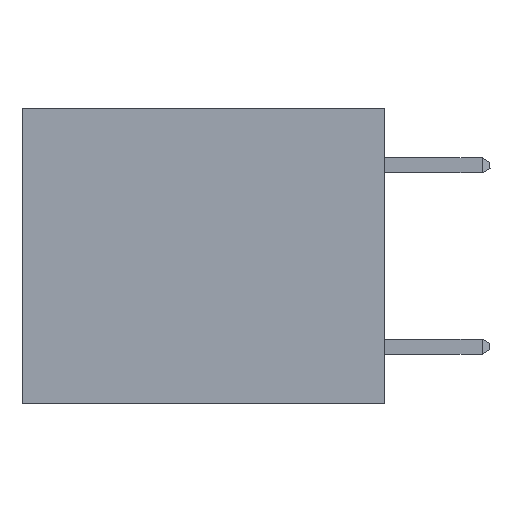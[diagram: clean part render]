
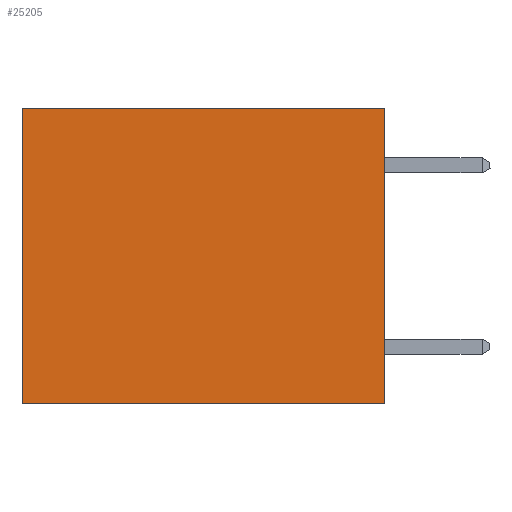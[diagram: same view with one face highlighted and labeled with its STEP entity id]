
A CAD part, left-side view. The second image highlights one B-rep face of the part: STEP entity #25205.
In plain terms, the highlighted planar face has unit normal (-1, 0, 0).
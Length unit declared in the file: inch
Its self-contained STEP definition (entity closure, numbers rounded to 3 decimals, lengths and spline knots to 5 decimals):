
#821 = LINE ( 'NONE', #17745, #24701 ) ;
#902 = EDGE_CURVE ( 'NONE', #22420, #20149, #2987, .T. ) ;
#1377 = DIRECTION ( 'NONE',  ( 0., 0., -1. ) ) ;
#2313 = VERTEX_POINT ( 'NONE', #26707 ) ;
#2987 = LINE ( 'NONE', #20899, #4164 ) ;
#4164 = VECTOR ( 'NONE', #8622, 39.37008 ) ;
#4547 = ORIENTED_EDGE ( 'NONE', *, *, #7767, .F. ) ;
#4949 = DIRECTION ( 'NONE',  ( 0., 1., 0. ) ) ;
#5919 = EDGE_LOOP ( 'NONE', ( #26563, #4547, #26533, #12764 ) ) ;
#7767 = EDGE_CURVE ( 'NONE', #22263, #20149, #821, .T. ) ;
#8622 = DIRECTION ( 'NONE',  ( 0., 0., -1. ) ) ;
#8946 = DIRECTION ( 'NONE',  ( 1., 0., 0. ) ) ;
#11538 = PLANE ( 'NONE',  #18131 ) ;
#12523 = CARTESIAN_POINT ( 'NONE',  ( 0.3165, 0.6, -0.49 ) ) ;
#12764 = ORIENTED_EDGE ( 'NONE', *, *, #16575, .T. ) ;
#15285 = VECTOR ( 'NONE', #17330, 39.37008 ) ;
#15567 = CARTESIAN_POINT ( 'NONE',  ( 0.3165, 0.6, 0. ) ) ;
#16575 = EDGE_CURVE ( 'NONE', #2313, #22420, #24248, .T. ) ;
#17330 = DIRECTION ( 'NONE',  ( 0., 0., -1. ) ) ;
#17742 = VECTOR ( 'NONE', #4949, 39.37008 ) ;
#17745 = CARTESIAN_POINT ( 'NONE',  ( 0.3165, 0., -0.49 ) ) ;
#18131 = AXIS2_PLACEMENT_3D ( 'NONE', #23652, #8946, #1377 ) ;
#18734 = CARTESIAN_POINT ( 'NONE',  ( 0.3165, 0., -0.49 ) ) ;
#19550 = CARTESIAN_POINT ( 'NONE',  ( 0.3165, 0., 0. ) ) ;
#20149 = VERTEX_POINT ( 'NONE', #12523 ) ;
#20214 = DIRECTION ( 'NONE',  ( 0., 1., 0. ) ) ;
#20874 = EDGE_CURVE ( 'NONE', #2313, #22263, #23326, .T. ) ;
#20899 = CARTESIAN_POINT ( 'NONE',  ( 0.3165, 0.6, -0.49 ) ) ;
#21572 = FACE_OUTER_BOUND ( 'NONE', #5919, .T. ) ;
#22263 = VERTEX_POINT ( 'NONE', #18734 ) ;
#22420 = VERTEX_POINT ( 'NONE', #15567 ) ;
#23326 = LINE ( 'NONE', #31645, #15285 ) ;
#23652 = CARTESIAN_POINT ( 'NONE',  ( 0.3165, 0., -0.49 ) ) ;
#24248 = LINE ( 'NONE', #19550, #17742 ) ;
#24701 = VECTOR ( 'NONE', #20214, 39.37008 ) ;
#25205 = ADVANCED_FACE ( 'NONE', ( #21572 ), #11538, .F. ) ;
#26533 = ORIENTED_EDGE ( 'NONE', *, *, #20874, .F. ) ;
#26563 = ORIENTED_EDGE ( 'NONE', *, *, #902, .T. ) ;
#26707 = CARTESIAN_POINT ( 'NONE',  ( 0.3165, 0., 0. ) ) ;
#31645 = CARTESIAN_POINT ( 'NONE',  ( 0.3165, 0., -0.49 ) ) ;
